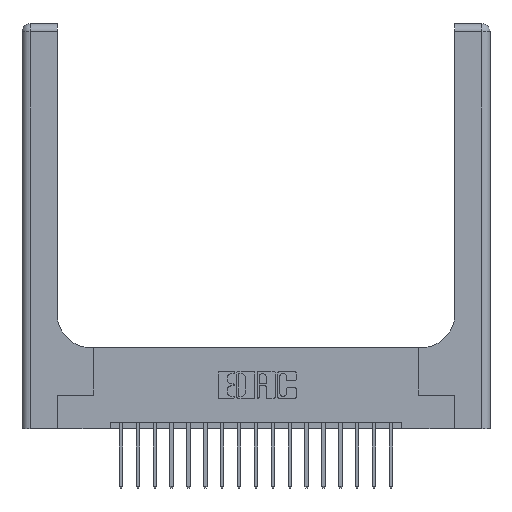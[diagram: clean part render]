
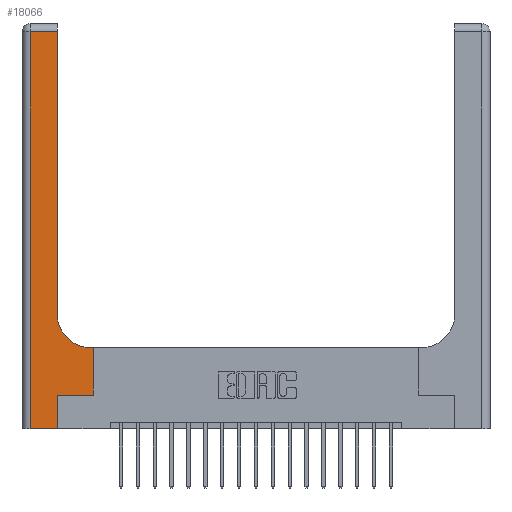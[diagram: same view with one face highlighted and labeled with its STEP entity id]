
A CAD part, top view. The second image highlights one B-rep face of the part: STEP entity #18066.
In plain terms, the highlighted planar face has unit normal (0, 0, 1).
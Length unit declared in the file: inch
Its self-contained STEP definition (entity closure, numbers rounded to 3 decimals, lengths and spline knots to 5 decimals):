
#299 = CARTESIAN_POINT ( 'NONE',  ( 0.26, 0.6, 0.37 ) ) ;
#312 = AXIS2_PLACEMENT_3D ( 'NONE', #18853, #17022, #6450 ) ;
#567 = VECTOR ( 'NONE', #3063, 39.37008 ) ;
#916 = CARTESIAN_POINT ( 'NONE',  ( 0.06, 0., 0.37 ) ) ;
#1429 = DIRECTION ( 'NONE',  ( -1., 0., 0. ) ) ;
#1457 = VECTOR ( 'NONE', #12537, 39.37008 ) ;
#1490 = EDGE_CURVE ( 'NONE', #14791, #13968, #9197, .T. ) ;
#1543 = LINE ( 'NONE', #17191, #567 ) ;
#1737 = EDGE_CURVE ( 'NONE', #17817, #10707, #1543, .T. ) ;
#2056 = LINE ( 'NONE', #11146, #14529 ) ;
#2125 = CARTESIAN_POINT ( 'NONE',  ( 0.26, 2.94, 0.37 ) ) ;
#2284 = LINE ( 'NONE', #7077, #7255 ) ;
#2417 = CARTESIAN_POINT ( 'NONE',  ( 0., 0., 0.37 ) ) ;
#2569 = CIRCLE ( 'NONE', #312, 0.25 ) ;
#2970 = VERTEX_POINT ( 'NONE', #16313 ) ;
#3063 = DIRECTION ( 'NONE',  ( 0., 1., 0. ) ) ;
#3135 = EDGE_CURVE ( 'NONE', #6258, #2970, #2569, .T. ) ;
#3480 = EDGE_CURVE ( 'NONE', #2970, #14377, #15461, .T. ) ;
#3856 = ORIENTED_EDGE ( 'NONE', *, *, #1737, .T. ) ;
#5264 = EDGE_CURVE ( 'NONE', #13968, #17817, #2284, .T. ) ;
#5516 = ORIENTED_EDGE ( 'NONE', *, *, #5729, .T. ) ;
#5706 = VECTOR ( 'NONE', #7120, 39.37008 ) ;
#5729 = EDGE_CURVE ( 'NONE', #10707, #6258, #6305, .T. ) ;
#6258 = VERTEX_POINT ( 'NONE', #17247 ) ;
#6304 = DIRECTION ( 'NONE',  ( 0., 1., 0. ) ) ;
#6305 = LINE ( 'NONE', #299, #1457 ) ;
#6414 = CARTESIAN_POINT ( 'NONE',  ( 0., 3., 0.37 ) ) ;
#6450 = DIRECTION ( 'NONE',  ( 1., 0., 0. ) ) ;
#6455 = DIRECTION ( 'NONE',  ( 0., -1., 0. ) ) ;
#6632 = ORIENTED_EDGE ( 'NONE', *, *, #16483, .T. ) ;
#6795 = EDGE_CURVE ( 'NONE', #18983, #9701, #2056, .T. ) ;
#7077 = CARTESIAN_POINT ( 'NONE',  ( 0.265, 0.25, 0.37 ) ) ;
#7120 = DIRECTION ( 'NONE',  ( 1., 0., 0. ) ) ;
#7255 = VECTOR ( 'NONE', #10230, 39.37008 ) ;
#7268 = CARTESIAN_POINT ( 'NONE',  ( 0., 2.94, 0.37 ) ) ;
#7355 = VECTOR ( 'NONE', #16820, 39.37008 ) ;
#7633 = FACE_OUTER_BOUND ( 'NONE', #15995, .T. ) ;
#7837 = CARTESIAN_POINT ( 'NONE',  ( 0.26, 3., 0.37 ) ) ;
#8043 = ORIENTED_EDGE ( 'NONE', *, *, #5264, .T. ) ;
#8423 = ORIENTED_EDGE ( 'NONE', *, *, #3135, .T. ) ;
#9047 = CARTESIAN_POINT ( 'NONE',  ( 0.528, 0.6, 0.37 ) ) ;
#9096 = DIRECTION ( 'NONE',  ( 0., 1., 0. ) ) ;
#9197 = LINE ( 'NONE', #11863, #11565 ) ;
#9687 = CARTESIAN_POINT ( 'NONE',  ( 0.528, 0.25, 0.37 ) ) ;
#9701 = VERTEX_POINT ( 'NONE', #916 ) ;
#10230 = DIRECTION ( 'NONE',  ( 1., 0., 0. ) ) ;
#10707 = VERTEX_POINT ( 'NONE', #9047 ) ;
#11146 = CARTESIAN_POINT ( 'NONE',  ( 0.06, 3., 0.37 ) ) ;
#11565 = VECTOR ( 'NONE', #9096, 39.37008 ) ;
#11863 = CARTESIAN_POINT ( 'NONE',  ( 0.265, 0., 0.37 ) ) ;
#11970 = CARTESIAN_POINT ( 'NONE',  ( 0.265, 0., 0.37 ) ) ;
#12349 = DIRECTION ( 'NONE',  ( 0., 0., -1. ) ) ;
#12537 = DIRECTION ( 'NONE',  ( -1., 0., 0. ) ) ;
#12752 = ORIENTED_EDGE ( 'NONE', *, *, #1490, .T. ) ;
#13656 = ORIENTED_EDGE ( 'NONE', *, *, #3480, .T. ) ;
#13968 = VERTEX_POINT ( 'NONE', #14362 ) ;
#14362 = CARTESIAN_POINT ( 'NONE',  ( 0.265, 0.25, 0.37 ) ) ;
#14377 = VERTEX_POINT ( 'NONE', #2125 ) ;
#14529 = VECTOR ( 'NONE', #6455, 39.37008 ) ;
#14791 = VERTEX_POINT ( 'NONE', #11970 ) ;
#14855 = AXIS2_PLACEMENT_3D ( 'NONE', #6414, #12349, #1429 ) ;
#14989 = LINE ( 'NONE', #7268, #7355 ) ;
#15461 = LINE ( 'NONE', #7837, #17536 ) ;
#15518 = ORIENTED_EDGE ( 'NONE', *, *, #15740, .T. ) ;
#15740 = EDGE_CURVE ( 'NONE', #9701, #14791, #16365, .T. ) ;
#15995 = EDGE_LOOP ( 'NONE', ( #13656, #6632, #20057, #15518, #12752, #8043, #3856, #5516, #8423 ) ) ;
#16313 = CARTESIAN_POINT ( 'NONE',  ( 0.26, 0.85, 0.37 ) ) ;
#16365 = LINE ( 'NONE', #2417, #5706 ) ;
#16483 = EDGE_CURVE ( 'NONE', #14377, #18983, #14989, .T. ) ;
#16820 = DIRECTION ( 'NONE',  ( -1., 0., 0. ) ) ;
#16938 = CARTESIAN_POINT ( 'NONE',  ( 0.06, 2.94, 0.37 ) ) ;
#17022 = DIRECTION ( 'NONE',  ( 0., 0., -1. ) ) ;
#17191 = CARTESIAN_POINT ( 'NONE',  ( 0.528, 0.25, 0.37 ) ) ;
#17247 = CARTESIAN_POINT ( 'NONE',  ( 0.51, 0.6, 0.37 ) ) ;
#17536 = VECTOR ( 'NONE', #6304, 39.37008 ) ;
#17817 = VERTEX_POINT ( 'NONE', #9687 ) ;
#18066 = ADVANCED_FACE ( 'NONE', ( #7633 ), #20043, .F. ) ;
#18853 = CARTESIAN_POINT ( 'NONE',  ( 0.51, 0.85, 0.37 ) ) ;
#18983 = VERTEX_POINT ( 'NONE', #16938 ) ;
#20043 = PLANE ( 'NONE',  #14855 ) ;
#20057 = ORIENTED_EDGE ( 'NONE', *, *, #6795, .T. ) ;
